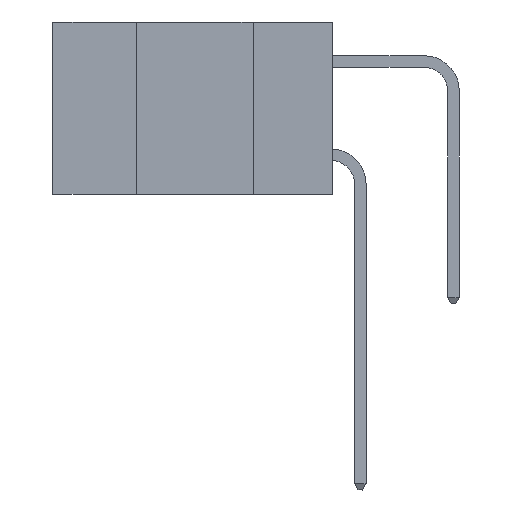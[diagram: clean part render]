
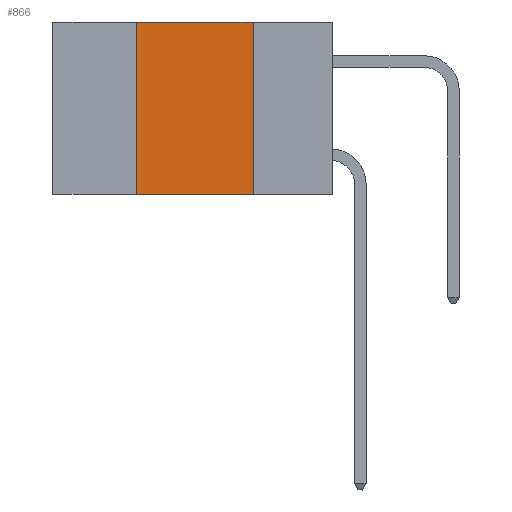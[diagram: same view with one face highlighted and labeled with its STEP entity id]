
A CAD part, left-side view. The second image highlights one B-rep face of the part: STEP entity #866.
In plain terms, the highlighted planar face has unit normal (-1, 0, 0).
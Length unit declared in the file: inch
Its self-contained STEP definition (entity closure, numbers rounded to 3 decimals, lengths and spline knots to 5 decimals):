
#866 = ADVANCED_FACE ( 'NONE', ( #10635 ), #11129, .F. ) ;
#940 = ORIENTED_EDGE ( 'NONE', *, *, #10856, .F. ) ;
#1348 = EDGE_CURVE ( 'NONE', #1915, #10806, #11987, .T. ) ;
#1915 = VERTEX_POINT ( 'NONE', #3760 ) ;
#2348 = EDGE_LOOP ( 'NONE', ( #940, #16408, #3057, #16560 ) ) ;
#2695 = DIRECTION ( 'NONE',  ( 1., 0., 0. ) ) ;
#3001 = DIRECTION ( 'NONE',  ( 0., 0., -1. ) ) ;
#3057 = ORIENTED_EDGE ( 'NONE', *, *, #15269, .F. ) ;
#3760 = CARTESIAN_POINT ( 'NONE',  ( 0., 0.42, -0.37 ) ) ;
#4289 = EDGE_CURVE ( 'NONE', #18665, #18138, #13460, .T. ) ;
#4970 = VECTOR ( 'NONE', #14908, 39.37008 ) ;
#5284 = CARTESIAN_POINT ( 'NONE',  ( 0., 0.6, 0. ) ) ;
#6249 = CARTESIAN_POINT ( 'NONE',  ( 0., 0.42, 0. ) ) ;
#6273 = CARTESIAN_POINT ( 'NONE',  ( 0., 0.17, 0. ) ) ;
#6615 = DIRECTION ( 'NONE',  ( 0., -1., 0. ) ) ;
#7312 = VECTOR ( 'NONE', #6615, 39.37008 ) ;
#7618 = DIRECTION ( 'NONE',  ( 0., 0., 1. ) ) ;
#8089 = VECTOR ( 'NONE', #15435, 39.37008 ) ;
#9845 = VECTOR ( 'NONE', #7618, 39.37008 ) ;
#10531 = AXIS2_PLACEMENT_3D ( 'NONE', #11397, #2695, #3001 ) ;
#10635 = FACE_OUTER_BOUND ( 'NONE', #2348, .T. ) ;
#10806 = VERTEX_POINT ( 'NONE', #12919 ) ;
#10856 = EDGE_CURVE ( 'NONE', #18138, #10806, #15864, .T. ) ;
#11129 = PLANE ( 'NONE',  #10531 ) ;
#11397 = CARTESIAN_POINT ( 'NONE',  ( 0., 0.6, 0. ) ) ;
#11987 = LINE ( 'NONE', #12540, #8089 ) ;
#12007 = CARTESIAN_POINT ( 'NONE',  ( 0., 0.17, 0. ) ) ;
#12540 = CARTESIAN_POINT ( 'NONE',  ( 0., 0.6, -0.37 ) ) ;
#12919 = CARTESIAN_POINT ( 'NONE',  ( 0., 0.17, -0.37 ) ) ;
#13460 = LINE ( 'NONE', #5284, #7312 ) ;
#14908 = DIRECTION ( 'NONE',  ( 0., 0., -1. ) ) ;
#15269 = EDGE_CURVE ( 'NONE', #1915, #18665, #17152, .T. ) ;
#15435 = DIRECTION ( 'NONE',  ( 0., -1., 0. ) ) ;
#15864 = LINE ( 'NONE', #12007, #4970 ) ;
#16408 = ORIENTED_EDGE ( 'NONE', *, *, #4289, .F. ) ;
#16560 = ORIENTED_EDGE ( 'NONE', *, *, #1348, .T. ) ;
#17152 = LINE ( 'NONE', #17774, #9845 ) ;
#17774 = CARTESIAN_POINT ( 'NONE',  ( 0., 0.42, 0. ) ) ;
#18138 = VERTEX_POINT ( 'NONE', #6273 ) ;
#18665 = VERTEX_POINT ( 'NONE', #6249 ) ;
